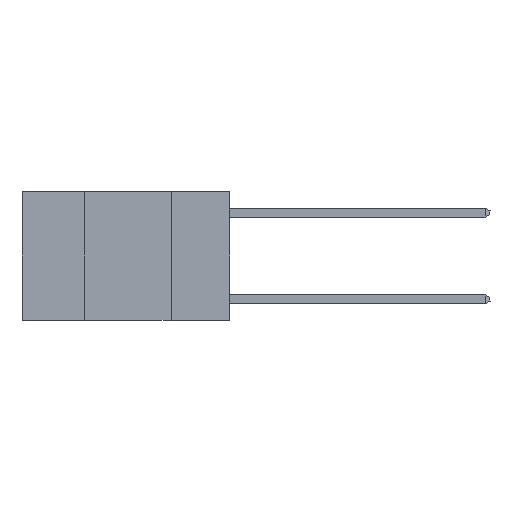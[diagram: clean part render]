
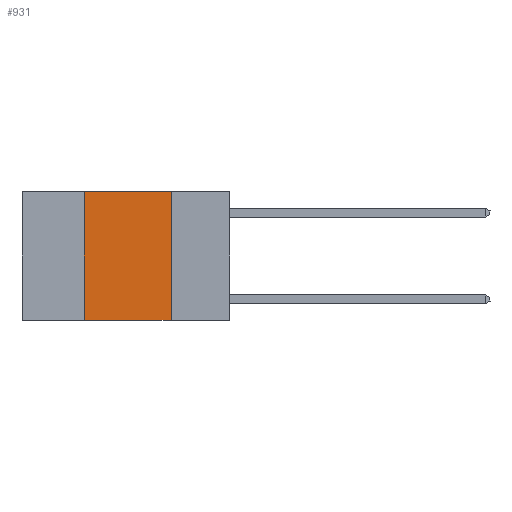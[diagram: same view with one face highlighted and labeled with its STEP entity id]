
A CAD part, left-side view. The second image highlights one B-rep face of the part: STEP entity #931.
In plain terms, the highlighted planar face has unit normal (-1, 0, 0).
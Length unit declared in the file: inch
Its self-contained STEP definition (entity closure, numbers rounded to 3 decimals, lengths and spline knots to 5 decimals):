
#125 = ORIENTED_EDGE ( 'NONE', *, *, #20655, .F. ) ;
#688 = DIRECTION ( 'NONE',  ( 0., -1., 0. ) ) ;
#792 = LINE ( 'NONE', #12597, #13804 ) ;
#931 = ADVANCED_FACE ( 'NONE', ( #10766 ), #7468, .F. ) ;
#1684 = VECTOR ( 'NONE', #688, 39.37008 ) ;
#1869 = VECTOR ( 'NONE', #19476, 39.37008 ) ;
#1972 = DIRECTION ( 'NONE',  ( 0., 0., 1. ) ) ;
#3495 = VERTEX_POINT ( 'NONE', #7058 ) ;
#3667 = EDGE_CURVE ( 'NONE', #3495, #19296, #14274, .T. ) ;
#3744 = VECTOR ( 'NONE', #1972, 39.37008 ) ;
#3980 = CARTESIAN_POINT ( 'NONE',  ( 0., 0.17, -0.37 ) ) ;
#4097 = CARTESIAN_POINT ( 'NONE',  ( 0., 0.6, 0. ) ) ;
#4701 = CARTESIAN_POINT ( 'NONE',  ( 0., 0.17, 0. ) ) ;
#5872 = DIRECTION ( 'NONE',  ( 1., 0., 0. ) ) ;
#5911 = ORIENTED_EDGE ( 'NONE', *, *, #11999, .F. ) ;
#6183 = CARTESIAN_POINT ( 'NONE',  ( 0., 0.42, 0. ) ) ;
#6618 = AXIS2_PLACEMENT_3D ( 'NONE', #13955, #5872, #15647 ) ;
#7058 = CARTESIAN_POINT ( 'NONE',  ( 0., 0.42, -0.37 ) ) ;
#7468 = PLANE ( 'NONE',  #6618 ) ;
#8348 = EDGE_LOOP ( 'NONE', ( #125, #20905, #5911, #19059 ) ) ;
#9316 = VERTEX_POINT ( 'NONE', #4701 ) ;
#10365 = LINE ( 'NONE', #4097, #1684 ) ;
#10766 = FACE_OUTER_BOUND ( 'NONE', #8348, .T. ) ;
#10847 = EDGE_CURVE ( 'NONE', #11412, #9316, #10365, .T. ) ;
#11202 = CARTESIAN_POINT ( 'NONE',  ( 0., 0.6, -0.37 ) ) ;
#11412 = VERTEX_POINT ( 'NONE', #6183 ) ;
#11999 = EDGE_CURVE ( 'NONE', #3495, #11412, #14736, .T. ) ;
#12597 = CARTESIAN_POINT ( 'NONE',  ( 0., 0.17, 0. ) ) ;
#13804 = VECTOR ( 'NONE', #17892, 39.37008 ) ;
#13955 = CARTESIAN_POINT ( 'NONE',  ( 0., 0.6, 0. ) ) ;
#14274 = LINE ( 'NONE', #11202, #1869 ) ;
#14736 = LINE ( 'NONE', #16835, #3744 ) ;
#15647 = DIRECTION ( 'NONE',  ( 0., 0., -1. ) ) ;
#16835 = CARTESIAN_POINT ( 'NONE',  ( 0., 0.42, 0. ) ) ;
#17892 = DIRECTION ( 'NONE',  ( 0., 0., -1. ) ) ;
#19059 = ORIENTED_EDGE ( 'NONE', *, *, #3667, .T. ) ;
#19296 = VERTEX_POINT ( 'NONE', #3980 ) ;
#19476 = DIRECTION ( 'NONE',  ( 0., -1., 0. ) ) ;
#20655 = EDGE_CURVE ( 'NONE', #9316, #19296, #792, .T. ) ;
#20905 = ORIENTED_EDGE ( 'NONE', *, *, #10847, .F. ) ;
